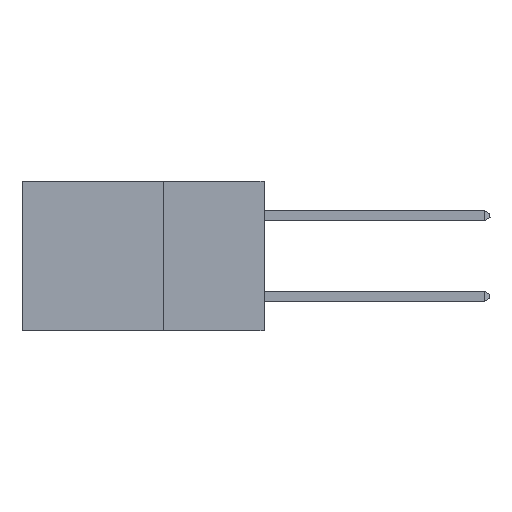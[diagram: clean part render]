
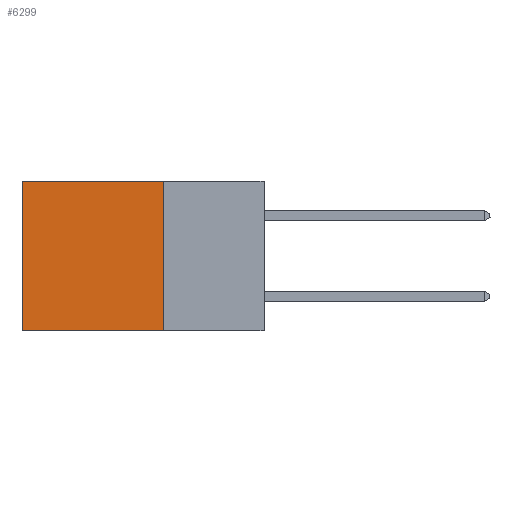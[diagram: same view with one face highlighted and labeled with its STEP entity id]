
A CAD part, left-side view. The second image highlights one B-rep face of the part: STEP entity #6299.
In plain terms, the highlighted planar face has unit normal (-1, 0, 0).
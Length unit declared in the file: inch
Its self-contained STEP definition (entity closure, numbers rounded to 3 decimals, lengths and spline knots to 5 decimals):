
#6 = LINE ( 'NONE', #5201, #20762 ) ;
#622 = EDGE_LOOP ( 'NONE', ( #3444, #10501, #5751, #7829 ) ) ;
#2802 = DIRECTION ( 'NONE',  ( 0., 0., -1. ) ) ;
#2860 = CARTESIAN_POINT ( 'NONE',  ( 0.298, 0.25, -0.37 ) ) ;
#3444 = ORIENTED_EDGE ( 'NONE', *, *, #17525, .T. ) ;
#3924 = PLANE ( 'NONE',  #4022 ) ;
#4022 = AXIS2_PLACEMENT_3D ( 'NONE', #9805, #20048, #23855 ) ;
#4155 = VERTEX_POINT ( 'NONE', #2860 ) ;
#4881 = CARTESIAN_POINT ( 'NONE',  ( 0.298, 0.25, 0. ) ) ;
#5201 = CARTESIAN_POINT ( 'NONE',  ( 0.298, 0.6, 0. ) ) ;
#5751 = ORIENTED_EDGE ( 'NONE', *, *, #7554, .F. ) ;
#6299 = ADVANCED_FACE ( 'NONE', ( #10814 ), #3924, .F. ) ;
#7147 = VERTEX_POINT ( 'NONE', #7863 ) ;
#7554 = EDGE_CURVE ( 'NONE', #16135, #4155, #20215, .T. ) ;
#7662 = CARTESIAN_POINT ( 'NONE',  ( 0.298, 0.25, 0. ) ) ;
#7829 = ORIENTED_EDGE ( 'NONE', *, *, #22555, .T. ) ;
#7863 = CARTESIAN_POINT ( 'NONE',  ( 0.298, 0.6, 0. ) ) ;
#9793 = EDGE_CURVE ( 'NONE', #4155, #20361, #13803, .T. ) ;
#9805 = CARTESIAN_POINT ( 'NONE',  ( 0.298, 0.25, 0. ) ) ;
#10501 = ORIENTED_EDGE ( 'NONE', *, *, #9793, .F. ) ;
#10814 = FACE_OUTER_BOUND ( 'NONE', #622, .T. ) ;
#10938 = VECTOR ( 'NONE', #17011, 39.37008 ) ;
#11124 = DIRECTION ( 'NONE',  ( 0., 1., 0. ) ) ;
#11643 = LINE ( 'NONE', #4881, #17321 ) ;
#13803 = LINE ( 'NONE', #23291, #10938 ) ;
#16135 = VERTEX_POINT ( 'NONE', #21206 ) ;
#17011 = DIRECTION ( 'NONE',  ( 0., 1., 0. ) ) ;
#17321 = VECTOR ( 'NONE', #11124, 39.37008 ) ;
#17525 = EDGE_CURVE ( 'NONE', #7147, #20361, #6, .T. ) ;
#17725 = VECTOR ( 'NONE', #21828, 39.37008 ) ;
#20048 = DIRECTION ( 'NONE',  ( 1., 0., 0. ) ) ;
#20215 = LINE ( 'NONE', #7662, #17725 ) ;
#20361 = VERTEX_POINT ( 'NONE', #20996 ) ;
#20762 = VECTOR ( 'NONE', #2802, 39.37008 ) ;
#20996 = CARTESIAN_POINT ( 'NONE',  ( 0.298, 0.6, -0.37 ) ) ;
#21206 = CARTESIAN_POINT ( 'NONE',  ( 0.298, 0.25, 0. ) ) ;
#21828 = DIRECTION ( 'NONE',  ( 0., 0., -1. ) ) ;
#22555 = EDGE_CURVE ( 'NONE', #16135, #7147, #11643, .T. ) ;
#23291 = CARTESIAN_POINT ( 'NONE',  ( 0.298, 0.25, -0.37 ) ) ;
#23855 = DIRECTION ( 'NONE',  ( 0., 0., -1. ) ) ;
